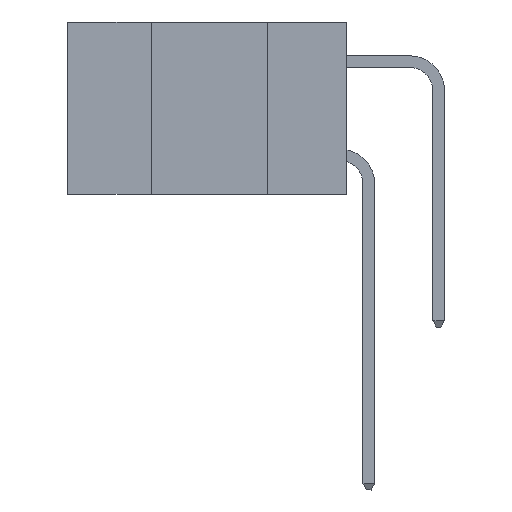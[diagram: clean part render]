
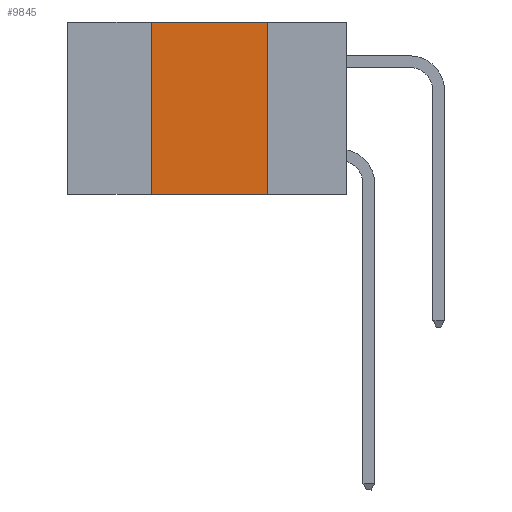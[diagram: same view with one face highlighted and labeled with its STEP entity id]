
A CAD part, left-side view. The second image highlights one B-rep face of the part: STEP entity #9845.
In plain terms, the highlighted planar face has unit normal (-1, 0, 0).
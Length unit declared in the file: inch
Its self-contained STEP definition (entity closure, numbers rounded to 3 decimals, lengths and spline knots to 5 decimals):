
#224 = VERTEX_POINT ( 'NONE', #901 ) ;
#373 = CARTESIAN_POINT ( 'NONE',  ( 0., 0.6, 0. ) ) ;
#534 = ORIENTED_EDGE ( 'NONE', *, *, #3596, .F. ) ;
#682 = VECTOR ( 'NONE', #3869, 39.37008 ) ;
#901 = CARTESIAN_POINT ( 'NONE',  ( 0., 0.42, -0.37 ) ) ;
#937 = DIRECTION ( 'NONE',  ( 0., 0., 1. ) ) ;
#1163 = ORIENTED_EDGE ( 'NONE', *, *, #3458, .F. ) ;
#1381 = VECTOR ( 'NONE', #937, 39.37008 ) ;
#2050 = FACE_OUTER_BOUND ( 'NONE', #10450, .T. ) ;
#2950 = CARTESIAN_POINT ( 'NONE',  ( 0., 0.6, 0. ) ) ;
#2963 = DIRECTION ( 'NONE',  ( 0., 0., -1. ) ) ;
#3331 = VERTEX_POINT ( 'NONE', #8469 ) ;
#3458 = EDGE_CURVE ( 'NONE', #224, #3331, #5212, .T. ) ;
#3596 = EDGE_CURVE ( 'NONE', #3331, #8615, #10706, .T. ) ;
#3869 = DIRECTION ( 'NONE',  ( 0., 0., -1. ) ) ;
#4104 = CARTESIAN_POINT ( 'NONE',  ( 0., 0.17, -0.37 ) ) ;
#4243 = DIRECTION ( 'NONE',  ( 0., -1., 0. ) ) ;
#4655 = CARTESIAN_POINT ( 'NONE',  ( 0., 0.17, 0. ) ) ;
#5153 = VECTOR ( 'NONE', #7169, 39.37008 ) ;
#5212 = LINE ( 'NONE', #8642, #1381 ) ;
#5751 = CARTESIAN_POINT ( 'NONE',  ( 0., 0.6, -0.37 ) ) ;
#6429 = CARTESIAN_POINT ( 'NONE',  ( 0., 0.17, 0. ) ) ;
#7169 = DIRECTION ( 'NONE',  ( 0., -1., 0. ) ) ;
#7499 = EDGE_CURVE ( 'NONE', #224, #8321, #10876, .T. ) ;
#7732 = VECTOR ( 'NONE', #4243, 39.37008 ) ;
#8078 = LINE ( 'NONE', #4655, #682 ) ;
#8080 = DIRECTION ( 'NONE',  ( 1., 0., 0. ) ) ;
#8321 = VERTEX_POINT ( 'NONE', #4104 ) ;
#8469 = CARTESIAN_POINT ( 'NONE',  ( 0., 0.42, 0. ) ) ;
#8615 = VERTEX_POINT ( 'NONE', #6429 ) ;
#8642 = CARTESIAN_POINT ( 'NONE',  ( 0., 0.42, 0. ) ) ;
#9050 = ORIENTED_EDGE ( 'NONE', *, *, #7499, .T. ) ;
#9845 = ADVANCED_FACE ( 'NONE', ( #2050 ), #10491, .F. ) ;
#10450 = EDGE_LOOP ( 'NONE', ( #11088, #534, #1163, #9050 ) ) ;
#10491 = PLANE ( 'NONE',  #10907 ) ;
#10706 = LINE ( 'NONE', #2950, #5153 ) ;
#10876 = LINE ( 'NONE', #5751, #7732 ) ;
#10907 = AXIS2_PLACEMENT_3D ( 'NONE', #373, #8080, #2963 ) ;
#11021 = EDGE_CURVE ( 'NONE', #8615, #8321, #8078, .T. ) ;
#11088 = ORIENTED_EDGE ( 'NONE', *, *, #11021, .F. ) ;
